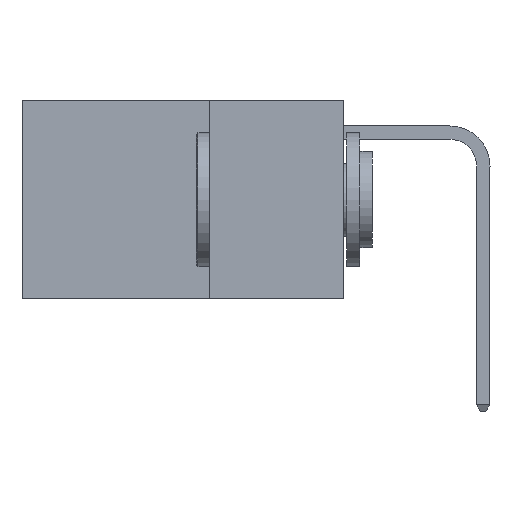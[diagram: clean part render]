
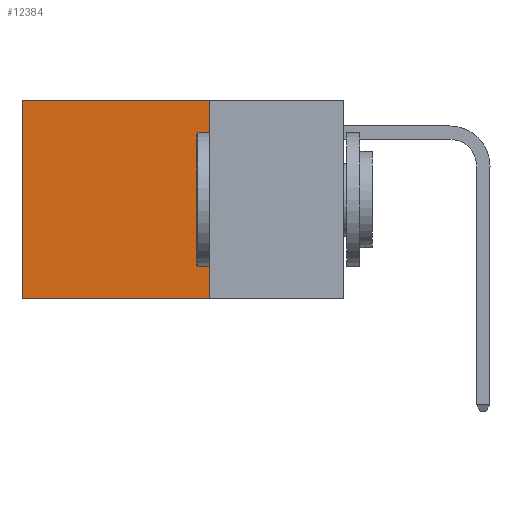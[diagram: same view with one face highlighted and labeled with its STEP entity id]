
A CAD part, left-side view. The second image highlights one B-rep face of the part: STEP entity #12384.
In plain terms, the highlighted planar face has unit normal (-1, 0, 0).
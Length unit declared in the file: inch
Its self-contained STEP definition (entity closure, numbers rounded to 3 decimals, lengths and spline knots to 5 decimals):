
#342 = AXIS2_PLACEMENT_3D ( 'NONE', #13664, #8763, #1263 ) ;
#417 = ORIENTED_EDGE ( 'NONE', *, *, #15824, .T. ) ;
#1263 = DIRECTION ( 'NONE',  ( 0., 0., -1. ) ) ;
#2355 = DIRECTION ( 'NONE',  ( 0., 1., 0. ) ) ;
#2800 = DIRECTION ( 'NONE',  ( 0., 0., -1. ) ) ;
#3021 = DIRECTION ( 'NONE',  ( 0., 1., 0. ) ) ;
#3748 = FACE_OUTER_BOUND ( 'NONE', #4358, .T. ) ;
#4358 = EDGE_LOOP ( 'NONE', ( #417, #10624, #5244, #9241 ) ) ;
#4715 = CARTESIAN_POINT ( 'NONE',  ( 0.2625, 0.6, 0. ) ) ;
#4860 = CARTESIAN_POINT ( 'NONE',  ( 0.2625, 0.25, 0. ) ) ;
#4969 = PLANE ( 'NONE',  #342 ) ;
#5244 = ORIENTED_EDGE ( 'NONE', *, *, #10749, .F. ) ;
#6104 = VECTOR ( 'NONE', #8500, 39.37008 ) ;
#6416 = VERTEX_POINT ( 'NONE', #10520 ) ;
#6494 = LINE ( 'NONE', #4715, #6104 ) ;
#7402 = VERTEX_POINT ( 'NONE', #12727 ) ;
#7474 = VECTOR ( 'NONE', #2355, 39.37008 ) ;
#8500 = DIRECTION ( 'NONE',  ( 0., 0., -1. ) ) ;
#8763 = DIRECTION ( 'NONE',  ( 1., 0., 0. ) ) ;
#8961 = EDGE_CURVE ( 'NONE', #10802, #15431, #13042, .T. ) ;
#8970 = CARTESIAN_POINT ( 'NONE',  ( 0.2625, 0.6, -0.37 ) ) ;
#9208 = CARTESIAN_POINT ( 'NONE',  ( 0.2625, 0.25, -0.37 ) ) ;
#9241 = ORIENTED_EDGE ( 'NONE', *, *, #12334, .T. ) ;
#9259 = CARTESIAN_POINT ( 'NONE',  ( 0.2625, 0.25, -0.37 ) ) ;
#9714 = VECTOR ( 'NONE', #3021, 39.37008 ) ;
#10290 = CARTESIAN_POINT ( 'NONE',  ( 0.2625, 0.25, 0. ) ) ;
#10520 = CARTESIAN_POINT ( 'NONE',  ( 0.2625, 0.25, 0. ) ) ;
#10624 = ORIENTED_EDGE ( 'NONE', *, *, #8961, .F. ) ;
#10749 = EDGE_CURVE ( 'NONE', #6416, #10802, #15706, .T. ) ;
#10802 = VERTEX_POINT ( 'NONE', #9208 ) ;
#12334 = EDGE_CURVE ( 'NONE', #6416, #7402, #14116, .T. ) ;
#12384 = ADVANCED_FACE ( 'NONE', ( #3748 ), #4969, .F. ) ;
#12412 = VECTOR ( 'NONE', #2800, 39.37008 ) ;
#12727 = CARTESIAN_POINT ( 'NONE',  ( 0.2625, 0.6, 0. ) ) ;
#13042 = LINE ( 'NONE', #9259, #9714 ) ;
#13664 = CARTESIAN_POINT ( 'NONE',  ( 0.2625, 0.25, 0. ) ) ;
#14116 = LINE ( 'NONE', #4860, #7474 ) ;
#15431 = VERTEX_POINT ( 'NONE', #8970 ) ;
#15706 = LINE ( 'NONE', #10290, #12412 ) ;
#15824 = EDGE_CURVE ( 'NONE', #7402, #15431, #6494, .T. ) ;
